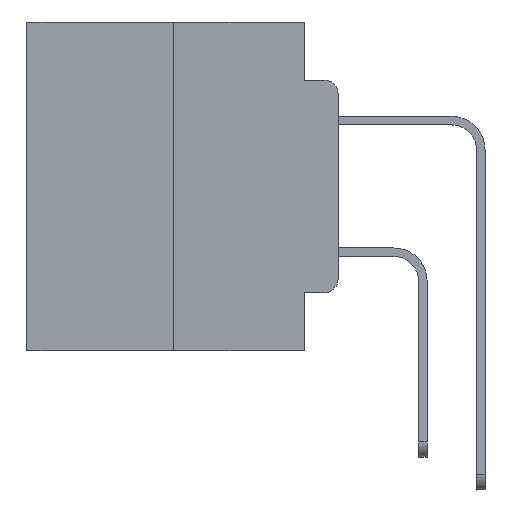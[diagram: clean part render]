
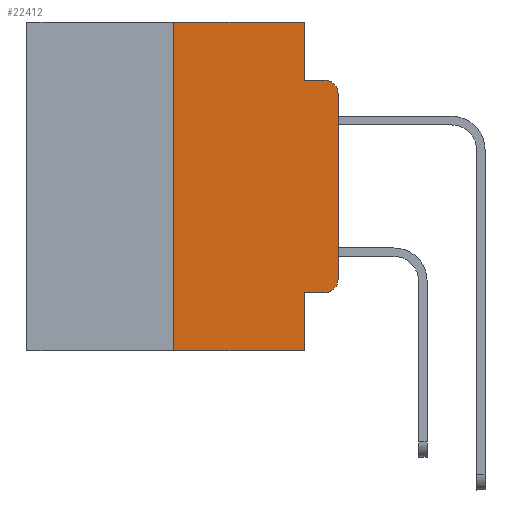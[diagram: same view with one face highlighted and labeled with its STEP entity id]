
A CAD part, left-side view. The second image highlights one B-rep face of the part: STEP entity #22412.
In plain terms, the highlighted planar face has unit normal (-1, 0, 0).
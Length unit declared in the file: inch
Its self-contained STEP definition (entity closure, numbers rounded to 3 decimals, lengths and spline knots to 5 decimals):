
#175 = DIRECTION ( 'NONE',  ( 0., 0., -1. ) ) ;
#1277 = CARTESIAN_POINT ( 'NONE',  ( 0., 0.473, -0.5 ) ) ;
#1280 = EDGE_CURVE ( 'NONE', #22447, #8918, #20367, .T. ) ;
#1341 = AXIS2_PLACEMENT_3D ( 'NONE', #16377, #18526, #5511 ) ;
#1608 = AXIS2_PLACEMENT_3D ( 'NONE', #2222, #17489, #4477 ) ;
#1883 = VERTEX_POINT ( 'NONE', #22235 ) ;
#1899 = LINE ( 'NONE', #7793, #18579 ) ;
#2222 = CARTESIAN_POINT ( 'NONE',  ( 0., 0.02, -0.1085 ) ) ;
#2984 = VECTOR ( 'NONE', #5509, 39.37008 ) ;
#3154 = EDGE_CURVE ( 'NONE', #25235, #18770, #1899, .T. ) ;
#3535 = CARTESIAN_POINT ( 'NONE',  ( 0., 0., 0. ) ) ;
#3567 = ORIENTED_EDGE ( 'NONE', *, *, #22799, .T. ) ;
#3798 = CARTESIAN_POINT ( 'NONE',  ( 0., 0.051, -0.5 ) ) ;
#4155 = CARTESIAN_POINT ( 'NONE',  ( 0., 0.051, -0.0885 ) ) ;
#4251 = VECTOR ( 'NONE', #7023, 39.37008 ) ;
#4477 = DIRECTION ( 'NONE',  ( 0., 0., -1. ) ) ;
#5229 = AXIS2_PLACEMENT_3D ( 'NONE', #26174, #13320, #175 ) ;
#5247 = ORIENTED_EDGE ( 'NONE', *, *, #8630, .T. ) ;
#5509 = DIRECTION ( 'NONE',  ( 0., 0., -1. ) ) ;
#5511 = DIRECTION ( 'NONE',  ( 0., 0., -1. ) ) ;
#5831 = VERTEX_POINT ( 'NONE', #21013 ) ;
#5832 = VERTEX_POINT ( 'NONE', #25274 ) ;
#6124 = LINE ( 'NONE', #8771, #17697 ) ;
#7023 = DIRECTION ( 'NONE',  ( 0., 0., 1. ) ) ;
#7638 = PLANE ( 'NONE',  #1341 ) ;
#7758 = DIRECTION ( 'NONE',  ( 0., 0., -1. ) ) ;
#7793 = CARTESIAN_POINT ( 'NONE',  ( 0., 0.051, 0. ) ) ;
#7882 = VECTOR ( 'NONE', #23063, 39.37008 ) ;
#8630 = EDGE_CURVE ( 'NONE', #1883, #18770, #19422, .T. ) ;
#8769 = VERTEX_POINT ( 'NONE', #27777 ) ;
#8771 = CARTESIAN_POINT ( 'NONE',  ( 0., 0.051, -0.4115 ) ) ;
#8918 = VERTEX_POINT ( 'NONE', #15425 ) ;
#9343 = CARTESIAN_POINT ( 'NONE',  ( 0., 0.051, 0. ) ) ;
#11432 = ORIENTED_EDGE ( 'NONE', *, *, #26199, .T. ) ;
#12013 = CARTESIAN_POINT ( 'NONE',  ( 0., 0.051, -0.4115 ) ) ;
#12770 = VECTOR ( 'NONE', #19341, 39.37008 ) ;
#12912 = LINE ( 'NONE', #13489, #23701 ) ;
#13320 = DIRECTION ( 'NONE',  ( -1., 0., 0. ) ) ;
#13333 = EDGE_CURVE ( 'NONE', #8769, #25482, #21119, .T. ) ;
#13489 = CARTESIAN_POINT ( 'NONE',  ( 0., 0.473, 0. ) ) ;
#13529 = FACE_OUTER_BOUND ( 'NONE', #23054, .T. ) ;
#13614 = ORIENTED_EDGE ( 'NONE', *, *, #23909, .F. ) ;
#14390 = DIRECTION ( 'NONE',  ( 0., 0., 1. ) ) ;
#14445 = LINE ( 'NONE', #20018, #4251 ) ;
#15358 = VECTOR ( 'NONE', #14390, 39.37008 ) ;
#15425 = CARTESIAN_POINT ( 'NONE',  ( 0., 0.051, -0.0885 ) ) ;
#15659 = DIRECTION ( 'NONE',  ( 0., -1., 0. ) ) ;
#15805 = ORIENTED_EDGE ( 'NONE', *, *, #28023, .T. ) ;
#16377 = CARTESIAN_POINT ( 'NONE',  ( 0., 0.473, 0. ) ) ;
#17238 = EDGE_CURVE ( 'NONE', #8918, #5832, #18488, .T. ) ;
#17489 = DIRECTION ( 'NONE',  ( -1., 0., 0. ) ) ;
#17697 = VECTOR ( 'NONE', #23889, 39.37008 ) ;
#18488 = LINE ( 'NONE', #4155, #12770 ) ;
#18526 = DIRECTION ( 'NONE',  ( 1., 0., 0. ) ) ;
#18579 = VECTOR ( 'NONE', #7758, 39.37008 ) ;
#18770 = VERTEX_POINT ( 'NONE', #3798 ) ;
#19341 = DIRECTION ( 'NONE',  ( 0., -1., 0. ) ) ;
#19422 = LINE ( 'NONE', #1277, #7882 ) ;
#20018 = CARTESIAN_POINT ( 'NONE',  ( 0., 0.25, 0. ) ) ;
#20101 = ORIENTED_EDGE ( 'NONE', *, *, #17238, .F. ) ;
#20367 = LINE ( 'NONE', #9343, #2984 ) ;
#20754 = VERTEX_POINT ( 'NONE', #21479 ) ;
#21013 = CARTESIAN_POINT ( 'NONE',  ( 0., 0.02, -0.4115 ) ) ;
#21119 = LINE ( 'NONE', #3535, #15358 ) ;
#21142 = ORIENTED_EDGE ( 'NONE', *, *, #21583, .F. ) ;
#21202 = CIRCLE ( 'NONE', #1608, 0.02 ) ;
#21479 = CARTESIAN_POINT ( 'NONE',  ( 0., 0.25, 0. ) ) ;
#21518 = ORIENTED_EDGE ( 'NONE', *, *, #1280, .F. ) ;
#21583 = EDGE_CURVE ( 'NONE', #20754, #22447, #12912, .T. ) ;
#22235 = CARTESIAN_POINT ( 'NONE',  ( 0., 0.25, -0.5 ) ) ;
#22412 = ADVANCED_FACE ( 'NONE', ( #13529 ), #7638, .F. ) ;
#22447 = VERTEX_POINT ( 'NONE', #22970 ) ;
#22799 = EDGE_CURVE ( 'NONE', #5831, #8769, #26262, .T. ) ;
#22970 = CARTESIAN_POINT ( 'NONE',  ( 0., 0.051, 0. ) ) ;
#23054 = EDGE_LOOP ( 'NONE', ( #26555, #11432, #20101, #21518, #21142, #13614, #5247, #26207, #15805, #3567 ) ) ;
#23063 = DIRECTION ( 'NONE',  ( 0., -1., 0. ) ) ;
#23701 = VECTOR ( 'NONE', #15659, 39.37008 ) ;
#23889 = DIRECTION ( 'NONE',  ( 0., -1., 0. ) ) ;
#23909 = EDGE_CURVE ( 'NONE', #1883, #20754, #14445, .T. ) ;
#25235 = VERTEX_POINT ( 'NONE', #12013 ) ;
#25274 = CARTESIAN_POINT ( 'NONE',  ( 0., 0.02, -0.0885 ) ) ;
#25482 = VERTEX_POINT ( 'NONE', #27840 ) ;
#26174 = CARTESIAN_POINT ( 'NONE',  ( 0., 0.02, -0.3915 ) ) ;
#26199 = EDGE_CURVE ( 'NONE', #25482, #5832, #21202, .T. ) ;
#26207 = ORIENTED_EDGE ( 'NONE', *, *, #3154, .F. ) ;
#26262 = CIRCLE ( 'NONE', #5229, 0.02 ) ;
#26555 = ORIENTED_EDGE ( 'NONE', *, *, #13333, .T. ) ;
#27777 = CARTESIAN_POINT ( 'NONE',  ( 0., 0., -0.3915 ) ) ;
#27840 = CARTESIAN_POINT ( 'NONE',  ( 0., 0., -0.1085 ) ) ;
#28023 = EDGE_CURVE ( 'NONE', #25235, #5831, #6124, .T. ) ;
